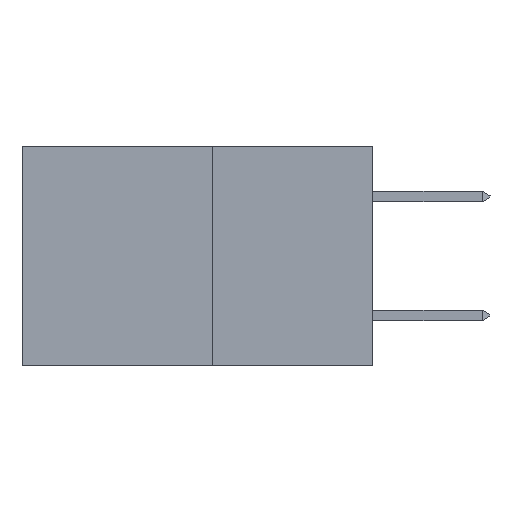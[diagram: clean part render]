
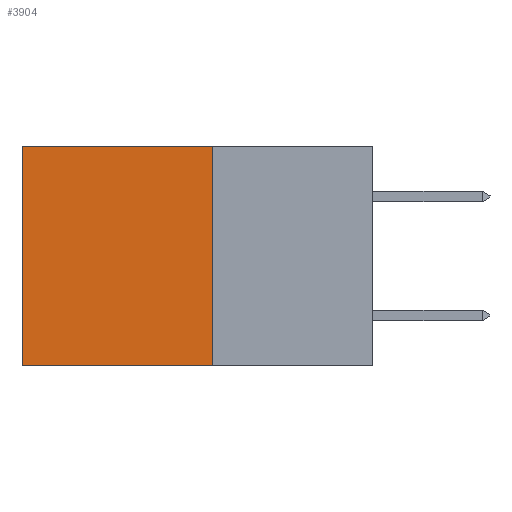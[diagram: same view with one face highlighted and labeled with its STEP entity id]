
A CAD part, left-side view. The second image highlights one B-rep face of the part: STEP entity #3904.
In plain terms, the highlighted planar face has unit normal (-1, 0, 0).
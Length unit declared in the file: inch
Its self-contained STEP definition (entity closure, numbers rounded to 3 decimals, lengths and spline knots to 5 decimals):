
#123 = LINE ( 'NONE', #553, #1769 ) ;
#331 = LINE ( 'NONE', #6330, #5237 ) ;
#553 = CARTESIAN_POINT ( 'NONE',  ( 0.277, 0.59, -0.37 ) ) ;
#736 = DIRECTION ( 'NONE',  ( 1., 0., 0. ) ) ;
#1111 = EDGE_LOOP ( 'NONE', ( #6202, #8105, #5226, #3259 ) ) ;
#1769 = VECTOR ( 'NONE', #4200, 39.37008 ) ;
#1869 = FACE_OUTER_BOUND ( 'NONE', #1111, .T. ) ;
#2136 = DIRECTION ( 'NONE',  ( 0., 0., -1. ) ) ;
#2765 = EDGE_CURVE ( 'NONE', #3713, #5163, #123, .T. ) ;
#2990 = CARTESIAN_POINT ( 'NONE',  ( 0.277, 0.27, 0. ) ) ;
#3029 = DIRECTION ( 'NONE',  ( 0., 1., 0. ) ) ;
#3259 = ORIENTED_EDGE ( 'NONE', *, *, #7693, .T. ) ;
#3644 = CARTESIAN_POINT ( 'NONE',  ( 0.277, 0.27, -0.37 ) ) ;
#3713 = VERTEX_POINT ( 'NONE', #6287 ) ;
#3904 = ADVANCED_FACE ( 'NONE', ( #1869 ), #5568, .F. ) ;
#4200 = DIRECTION ( 'NONE',  ( 0., 0., -1. ) ) ;
#4629 = LINE ( 'NONE', #7372, #5910 ) ;
#4673 = CARTESIAN_POINT ( 'NONE',  ( 0.277, 0.59, -0.37 ) ) ;
#4993 = EDGE_CURVE ( 'NONE', #7201, #5578, #331, .T. ) ;
#5163 = VERTEX_POINT ( 'NONE', #4673 ) ;
#5226 = ORIENTED_EDGE ( 'NONE', *, *, #4993, .F. ) ;
#5237 = VECTOR ( 'NONE', #6281, 39.37008 ) ;
#5568 = PLANE ( 'NONE',  #7853 ) ;
#5578 = VERTEX_POINT ( 'NONE', #8118 ) ;
#5910 = VECTOR ( 'NONE', #7446, 39.37008 ) ;
#6202 = ORIENTED_EDGE ( 'NONE', *, *, #2765, .T. ) ;
#6264 = VECTOR ( 'NONE', #3029, 39.37008 ) ;
#6281 = DIRECTION ( 'NONE',  ( 0., 0., -1. ) ) ;
#6287 = CARTESIAN_POINT ( 'NONE',  ( 0.277, 0.59, 0. ) ) ;
#6330 = CARTESIAN_POINT ( 'NONE',  ( 0.277, 0.27, -0.37 ) ) ;
#7201 = VERTEX_POINT ( 'NONE', #7681 ) ;
#7253 = EDGE_CURVE ( 'NONE', #5578, #5163, #4629, .T. ) ;
#7372 = CARTESIAN_POINT ( 'NONE',  ( 0.277, 0.27, -0.37 ) ) ;
#7446 = DIRECTION ( 'NONE',  ( 0., 1., 0. ) ) ;
#7681 = CARTESIAN_POINT ( 'NONE',  ( 0.277, 0.27, 0. ) ) ;
#7693 = EDGE_CURVE ( 'NONE', #7201, #3713, #7895, .T. ) ;
#7853 = AXIS2_PLACEMENT_3D ( 'NONE', #3644, #736, #2136 ) ;
#7895 = LINE ( 'NONE', #2990, #6264 ) ;
#8105 = ORIENTED_EDGE ( 'NONE', *, *, #7253, .F. ) ;
#8118 = CARTESIAN_POINT ( 'NONE',  ( 0.277, 0.27, -0.37 ) ) ;
